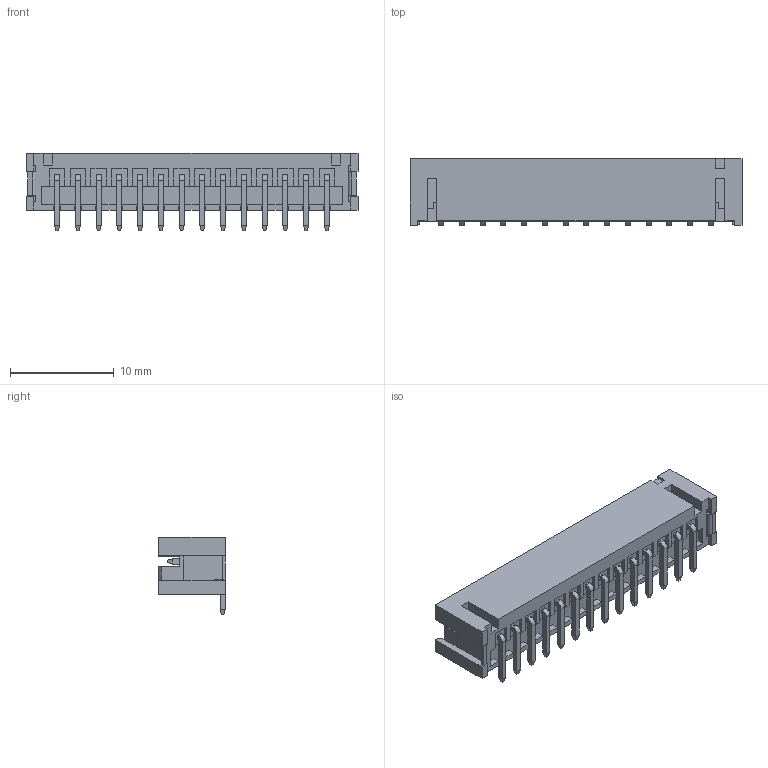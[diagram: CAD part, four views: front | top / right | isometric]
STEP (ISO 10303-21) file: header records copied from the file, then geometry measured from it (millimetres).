
FILE_DESCRIPTION (( 'STEP AP203' ), '1' );
FILE_NAME ('140-514-417-011.STEP', '2020-03-31T20:07:29', ( '' ), ( '' ), 'SwSTEP 2.0', 'SolidWorks 2016', '' );
FILE_SCHEMA (( 'CONFIG_CONTROL_DESIGN' ));
Length unit declared in the file: millimetre
Products named in the file (4): 140-514-417-011; V SMT Housing_514; V SMT Contact; V SMT Pad
Assembly tree (17 placements, depth 2):
  140-514-417-011
    V SMT Housing_514
    V SMT Contact  x14
    V SMT Pad  x2
Bounding box: 32 x 6.4 x 7.5 mm (x, y, z)
Volume: 454.5 mm3; surface area: 1648.3 mm2
Topology: 17 solids, 17 shells, 632 faces, 1572 edges, 970 vertices
Faces by surface type: plane 600, cylinder 32
Entity records: 11614 total; most frequent: CARTESIAN_POINT 1950, ORIENTED_EDGE 1928, DIRECTION 1676, EDGE_CURVE 964, VECTOR 956, LINE 956, VERTEX_POINT 634, EDGE_LOOP 360
